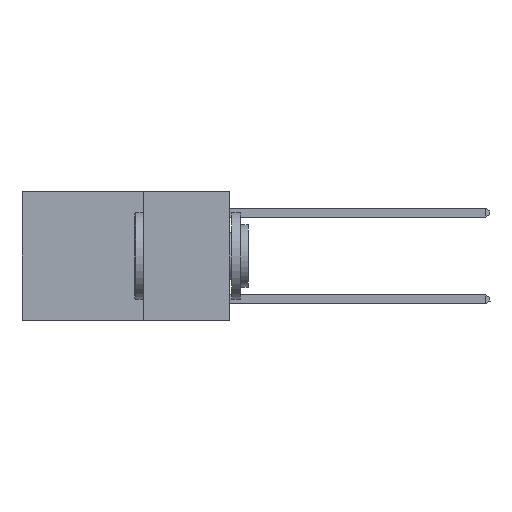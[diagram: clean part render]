
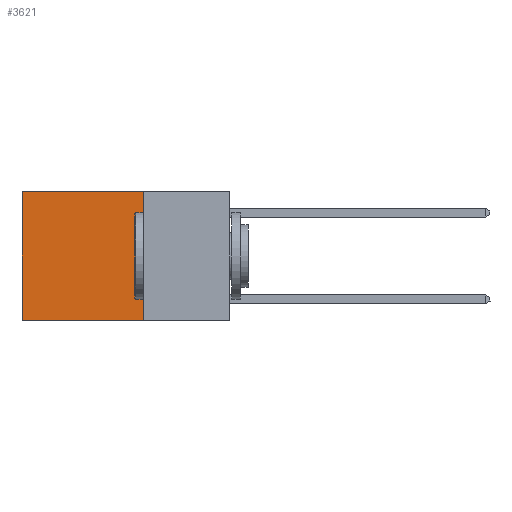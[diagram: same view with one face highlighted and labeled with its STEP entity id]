
A CAD part, left-side view. The second image highlights one B-rep face of the part: STEP entity #3621.
In plain terms, the highlighted planar face has unit normal (-1, 0, 0).
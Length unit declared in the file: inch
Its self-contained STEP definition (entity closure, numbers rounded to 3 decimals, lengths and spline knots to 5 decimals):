
#439 = AXIS2_PLACEMENT_3D ( 'NONE', #11812, #7935, #11340 ) ;
#601 = CARTESIAN_POINT ( 'NONE',  ( 0.2625, 0.25, 0. ) ) ;
#1123 = VERTEX_POINT ( 'NONE', #2022 ) ;
#1403 = VERTEX_POINT ( 'NONE', #601 ) ;
#1437 = DIRECTION ( 'NONE',  ( 0., 1., 0. ) ) ;
#1451 = EDGE_CURVE ( 'NONE', #1936, #10824, #7559, .T. ) ;
#1936 = VERTEX_POINT ( 'NONE', #11630 ) ;
#2022 = CARTESIAN_POINT ( 'NONE',  ( 0.2625, 0.6, 0. ) ) ;
#3073 = ORIENTED_EDGE ( 'NONE', *, *, #3782, .T. ) ;
#3344 = VECTOR ( 'NONE', #12560, 39.37008 ) ;
#3621 = ADVANCED_FACE ( 'NONE', ( #7498 ), #11523, .F. ) ;
#3782 = EDGE_CURVE ( 'NONE', #1403, #1123, #8696, .T. ) ;
#4011 = CARTESIAN_POINT ( 'NONE',  ( 0.2625, 0.25, 0. ) ) ;
#4346 = CARTESIAN_POINT ( 'NONE',  ( 0.2625, 0.25, -0.37 ) ) ;
#4402 = VECTOR ( 'NONE', #1437, 39.37008 ) ;
#4558 = ORIENTED_EDGE ( 'NONE', *, *, #11825, .F. ) ;
#5055 = DIRECTION ( 'NONE',  ( 0., 0., -1. ) ) ;
#6169 = CARTESIAN_POINT ( 'NONE',  ( 0.2625, 0.6, 0. ) ) ;
#7498 = FACE_OUTER_BOUND ( 'NONE', #11118, .T. ) ;
#7559 = LINE ( 'NONE', #4346, #4402 ) ;
#7935 = DIRECTION ( 'NONE',  ( 1., 0., 0. ) ) ;
#8076 = ORIENTED_EDGE ( 'NONE', *, *, #8892, .T. ) ;
#8106 = VECTOR ( 'NONE', #5055, 39.37008 ) ;
#8696 = LINE ( 'NONE', #12421, #3344 ) ;
#8892 = EDGE_CURVE ( 'NONE', #1123, #10824, #10039, .T. ) ;
#10039 = LINE ( 'NONE', #6169, #12433 ) ;
#10572 = ORIENTED_EDGE ( 'NONE', *, *, #1451, .F. ) ;
#10824 = VERTEX_POINT ( 'NONE', #12789 ) ;
#10908 = LINE ( 'NONE', #4011, #8106 ) ;
#11118 = EDGE_LOOP ( 'NONE', ( #8076, #10572, #4558, #3073 ) ) ;
#11340 = DIRECTION ( 'NONE',  ( 0., 0., -1. ) ) ;
#11523 = PLANE ( 'NONE',  #439 ) ;
#11630 = CARTESIAN_POINT ( 'NONE',  ( 0.2625, 0.25, -0.37 ) ) ;
#11812 = CARTESIAN_POINT ( 'NONE',  ( 0.2625, 0.25, 0. ) ) ;
#11825 = EDGE_CURVE ( 'NONE', #1403, #1936, #10908, .T. ) ;
#12421 = CARTESIAN_POINT ( 'NONE',  ( 0.2625, 0.25, 0. ) ) ;
#12433 = VECTOR ( 'NONE', #13426, 39.37008 ) ;
#12560 = DIRECTION ( 'NONE',  ( 0., 1., 0. ) ) ;
#12789 = CARTESIAN_POINT ( 'NONE',  ( 0.2625, 0.6, -0.37 ) ) ;
#13426 = DIRECTION ( 'NONE',  ( 0., 0., -1. ) ) ;
